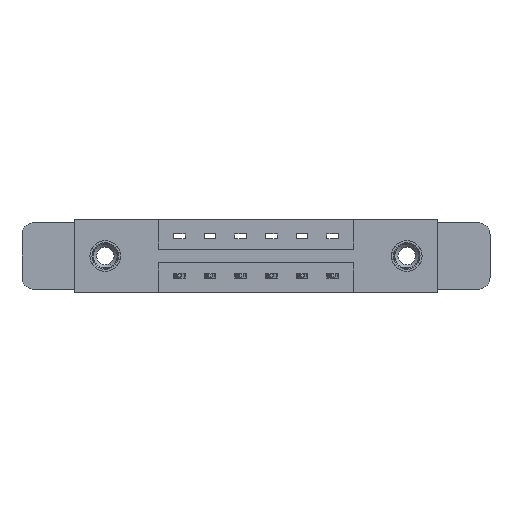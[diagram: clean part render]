
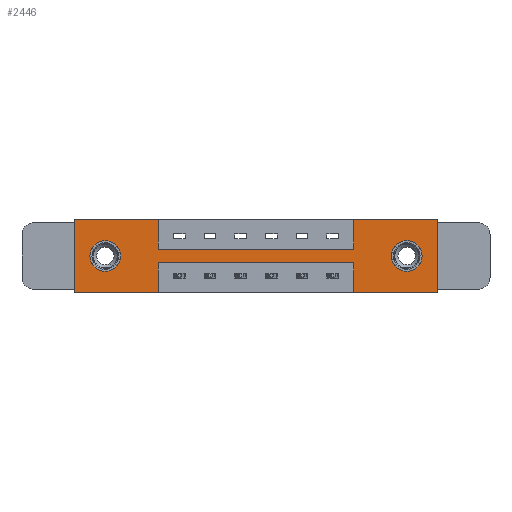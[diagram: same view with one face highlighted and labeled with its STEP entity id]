
A CAD part, front view. The second image highlights one B-rep face of the part: STEP entity #2446.
In plain terms, the highlighted planar face has unit normal (0, -1, 0).
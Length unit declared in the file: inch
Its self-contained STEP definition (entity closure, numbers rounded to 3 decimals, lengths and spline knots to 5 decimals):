
#35 = DIRECTION ( 'NONE',  ( 0., 1., 0. ) ) ;
#72 = CARTESIAN_POINT ( 'NONE',  ( 1.687, 0., -0.263 ) ) ;
#93 = ORIENTED_EDGE ( 'NONE', *, *, #8928, .F. ) ;
#447 = LINE ( 'NONE', #4689, #7954 ) ;
#464 = EDGE_CURVE ( 'NONE', #8278, #10195, #6132, .T. ) ;
#493 = CARTESIAN_POINT ( 'NONE',  ( 0.425, 0., 0. ) ) ;
#571 = CIRCLE ( 'NONE', #1085, 0.078 ) ;
#808 = LINE ( 'NONE', #3687, #4784 ) ;
#823 = ORIENTED_EDGE ( 'NONE', *, *, #11051, .F. ) ;
#857 = VERTEX_POINT ( 'NONE', #7307 ) ;
#1085 = AXIS2_PLACEMENT_3D ( 'NONE', #3840, #9292, #11082 ) ;
#1113 = CARTESIAN_POINT ( 'NONE',  ( 0., 0., 0. ) ) ;
#1230 = CARTESIAN_POINT ( 'NONE',  ( 0.155, 0., -0.107 ) ) ;
#1472 = ORIENTED_EDGE ( 'NONE', *, *, #464, .F. ) ;
#1555 = EDGE_CURVE ( 'NONE', #4462, #7166, #3856, .T. ) ;
#1600 = CARTESIAN_POINT ( 'NONE',  ( 1.417, 0., -0.15 ) ) ;
#1787 = ORIENTED_EDGE ( 'NONE', *, *, #2870, .T. ) ;
#2103 = CIRCLE ( 'NONE', #7834, 0.078 ) ;
#2293 = VECTOR ( 'NONE', #5236, 39.37008 ) ;
#2316 = CARTESIAN_POINT ( 'NONE',  ( 0.425, 0., -0.15 ) ) ;
#2446 = ADVANCED_FACE ( 'NONE', ( #9237, #8093, #8958 ), #11409, .T. ) ;
#2493 = CARTESIAN_POINT ( 'NONE',  ( 1.417, 0., -0.37 ) ) ;
#2511 = CARTESIAN_POINT ( 'NONE',  ( 0.425, 0., -0.37 ) ) ;
#2624 = EDGE_CURVE ( 'NONE', #10195, #3910, #10980, .T. ) ;
#2663 = CARTESIAN_POINT ( 'NONE',  ( 0.425, 0., 0. ) ) ;
#2870 = EDGE_CURVE ( 'NONE', #8690, #9549, #571, .T. ) ;
#2927 = VERTEX_POINT ( 'NONE', #8402 ) ;
#2949 = EDGE_LOOP ( 'NONE', ( #10601, #3054, #823, #3131, #5890, #1472, #8414, #6598, #2987, #8954, #4121, #93 ) ) ;
#2987 = ORIENTED_EDGE ( 'NONE', *, *, #10875, .F. ) ;
#3054 = ORIENTED_EDGE ( 'NONE', *, *, #5545, .F. ) ;
#3131 = ORIENTED_EDGE ( 'NONE', *, *, #8662, .F. ) ;
#3208 = DIRECTION ( 'NONE',  ( 0., 0., -1. ) ) ;
#3327 = VECTOR ( 'NONE', #5101, 39.37008 ) ;
#3341 = CARTESIAN_POINT ( 'NONE',  ( 0.425, 0., -0.37 ) ) ;
#3411 = LINE ( 'NONE', #2316, #7914 ) ;
#3439 = CARTESIAN_POINT ( 'NONE',  ( 0.425, 0., -0.15 ) ) ;
#3445 = EDGE_CURVE ( 'NONE', #4766, #3598, #3411, .T. ) ;
#3598 = VERTEX_POINT ( 'NONE', #1600 ) ;
#3615 = DIRECTION ( 'NONE',  ( 0., 0., 1. ) ) ;
#3654 = VERTEX_POINT ( 'NONE', #8764 ) ;
#3687 = CARTESIAN_POINT ( 'NONE',  ( 0.425, 0., -0.22 ) ) ;
#3840 = CARTESIAN_POINT ( 'NONE',  ( 1.687, 0., -0.185 ) ) ;
#3856 = LINE ( 'NONE', #11221, #5380 ) ;
#3910 = VERTEX_POINT ( 'NONE', #7349 ) ;
#4015 = CARTESIAN_POINT ( 'NONE',  ( 1.687, 0., -0.107 ) ) ;
#4121 = ORIENTED_EDGE ( 'NONE', *, *, #1555, .F. ) ;
#4282 = VECTOR ( 'NONE', #4962, 39.37008 ) ;
#4322 = CARTESIAN_POINT ( 'NONE',  ( 0., 0., 0. ) ) ;
#4343 = EDGE_LOOP ( 'NONE', ( #8923, #7472 ) ) ;
#4462 = VERTEX_POINT ( 'NONE', #9364 ) ;
#4470 = VERTEX_POINT ( 'NONE', #1230 ) ;
#4689 = CARTESIAN_POINT ( 'NONE',  ( 1.417, 0., 0. ) ) ;
#4701 = ORIENTED_EDGE ( 'NONE', *, *, #5756, .T. ) ;
#4766 = VERTEX_POINT ( 'NONE', #3439 ) ;
#4784 = VECTOR ( 'NONE', #6395, 39.37008 ) ;
#4912 = EDGE_LOOP ( 'NONE', ( #1787, #4701 ) ) ;
#4927 = DIRECTION ( 'NONE',  ( 0., 1., 0. ) ) ;
#4958 = VECTOR ( 'NONE', #11738, 39.37008 ) ;
#4962 = DIRECTION ( 'NONE',  ( 0., 0., -1. ) ) ;
#5101 = DIRECTION ( 'NONE',  ( 0., 0., -1. ) ) ;
#5236 = DIRECTION ( 'NONE',  ( 0., 0., 1. ) ) ;
#5293 = DIRECTION ( 'NONE',  ( 0., 1., 0. ) ) ;
#5358 = DIRECTION ( 'NONE',  ( 0., 0., 1. ) ) ;
#5380 = VECTOR ( 'NONE', #10156, 39.37008 ) ;
#5438 = CARTESIAN_POINT ( 'NONE',  ( 0., 0., -0.37 ) ) ;
#5545 = EDGE_CURVE ( 'NONE', #857, #2927, #808, .T. ) ;
#5616 = VERTEX_POINT ( 'NONE', #2663 ) ;
#5634 = EDGE_CURVE ( 'NONE', #7166, #5616, #11198, .T. ) ;
#5756 = EDGE_CURVE ( 'NONE', #9549, #8690, #8302, .T. ) ;
#5772 = AXIS2_PLACEMENT_3D ( 'NONE', #7779, #7730, #3208 ) ;
#5889 = DIRECTION ( 'NONE',  ( 1., 0., 0. ) ) ;
#5890 = ORIENTED_EDGE ( 'NONE', *, *, #2624, .F. ) ;
#6092 = DIRECTION ( 'NONE',  ( 1., 0., 0. ) ) ;
#6132 = LINE ( 'NONE', #1113, #7980 ) ;
#6280 = CARTESIAN_POINT ( 'NONE',  ( 1.417, 0., -0.37 ) ) ;
#6395 = DIRECTION ( 'NONE',  ( -1., 0., 0. ) ) ;
#6598 = ORIENTED_EDGE ( 'NONE', *, *, #3445, .F. ) ;
#6727 = VECTOR ( 'NONE', #9914, 39.37008 ) ;
#6730 = DIRECTION ( 'NONE',  ( 0., 0., -1. ) ) ;
#6945 = DIRECTION ( 'NONE',  ( 0., 0., -1. ) ) ;
#6949 = VECTOR ( 'NONE', #8556, 39.37008 ) ;
#7071 = CARTESIAN_POINT ( 'NONE',  ( 0.155, 0., -0.185 ) ) ;
#7165 = EDGE_CURVE ( 'NONE', #2927, #7195, #10871, .T. ) ;
#7166 = VERTEX_POINT ( 'NONE', #4322 ) ;
#7195 = VERTEX_POINT ( 'NONE', #3341 ) ;
#7307 = CARTESIAN_POINT ( 'NONE',  ( 1.417, 0., -0.22 ) ) ;
#7349 = CARTESIAN_POINT ( 'NONE',  ( 1.842, 0., -0.37 ) ) ;
#7472 = ORIENTED_EDGE ( 'NONE', *, *, #8976, .T. ) ;
#7638 = CIRCLE ( 'NONE', #10293, 0.078 ) ;
#7730 = DIRECTION ( 'NONE',  ( 0., -1., 0. ) ) ;
#7779 = CARTESIAN_POINT ( 'NONE',  ( 0., 0., -0.37 ) ) ;
#7834 = AXIS2_PLACEMENT_3D ( 'NONE', #9835, #35, #5358 ) ;
#7914 = VECTOR ( 'NONE', #5889, 39.37008 ) ;
#7954 = VECTOR ( 'NONE', #11074, 39.37008 ) ;
#7980 = VECTOR ( 'NONE', #6092, 39.37008 ) ;
#8091 = CARTESIAN_POINT ( 'NONE',  ( 1.417, 0., 0. ) ) ;
#8093 = FACE_BOUND ( 'NONE', #4343, .T. ) ;
#8278 = VERTEX_POINT ( 'NONE', #8091 ) ;
#8302 = CIRCLE ( 'NONE', #9651, 0.078 ) ;
#8402 = CARTESIAN_POINT ( 'NONE',  ( 0.425, 0., -0.22 ) ) ;
#8414 = ORIENTED_EDGE ( 'NONE', *, *, #8456, .F. ) ;
#8456 = EDGE_CURVE ( 'NONE', #3598, #8278, #447, .T. ) ;
#8556 = DIRECTION ( 'NONE',  ( -1., 0., 0. ) ) ;
#8582 = CARTESIAN_POINT ( 'NONE',  ( 1.842, 0., 0. ) ) ;
#8652 = LINE ( 'NONE', #5438, #4958 ) ;
#8662 = EDGE_CURVE ( 'NONE', #3910, #9005, #10377, .T. ) ;
#8690 = VERTEX_POINT ( 'NONE', #4015 ) ;
#8764 = CARTESIAN_POINT ( 'NONE',  ( 0.155, 0., -0.263 ) ) ;
#8923 = ORIENTED_EDGE ( 'NONE', *, *, #9440, .T. ) ;
#8928 = EDGE_CURVE ( 'NONE', #7195, #4462, #8652, .T. ) ;
#8945 = VECTOR ( 'NONE', #6945, 39.37008 ) ;
#8954 = ORIENTED_EDGE ( 'NONE', *, *, #5634, .F. ) ;
#8958 = FACE_OUTER_BOUND ( 'NONE', #2949, .T. ) ;
#8964 = LINE ( 'NONE', #493, #4282 ) ;
#8976 = EDGE_CURVE ( 'NONE', #3654, #4470, #7638, .T. ) ;
#9005 = VERTEX_POINT ( 'NONE', #6280 ) ;
#9237 = FACE_BOUND ( 'NONE', #4912, .T. ) ;
#9292 = DIRECTION ( 'NONE',  ( 0., 1., 0. ) ) ;
#9364 = CARTESIAN_POINT ( 'NONE',  ( 0., 0., -0.37 ) ) ;
#9440 = EDGE_CURVE ( 'NONE', #4470, #3654, #2103, .T. ) ;
#9549 = VERTEX_POINT ( 'NONE', #72 ) ;
#9651 = AXIS2_PLACEMENT_3D ( 'NONE', #11363, #4927, #6730 ) ;
#9739 = CARTESIAN_POINT ( 'NONE',  ( 1.842, 0., 0. ) ) ;
#9835 = CARTESIAN_POINT ( 'NONE',  ( 0.155, 0., -0.185 ) ) ;
#9914 = DIRECTION ( 'NONE',  ( 1., 0., 0. ) ) ;
#9959 = CARTESIAN_POINT ( 'NONE',  ( 0., 0., 0. ) ) ;
#10156 = DIRECTION ( 'NONE',  ( 0., 0., 1. ) ) ;
#10195 = VERTEX_POINT ( 'NONE', #8582 ) ;
#10293 = AXIS2_PLACEMENT_3D ( 'NONE', #7071, #5293, #3615 ) ;
#10377 = LINE ( 'NONE', #10487, #6949 ) ;
#10487 = CARTESIAN_POINT ( 'NONE',  ( 0., 0., -0.37 ) ) ;
#10601 = ORIENTED_EDGE ( 'NONE', *, *, #7165, .F. ) ;
#10871 = LINE ( 'NONE', #2511, #3327 ) ;
#10875 = EDGE_CURVE ( 'NONE', #5616, #4766, #8964, .T. ) ;
#10980 = LINE ( 'NONE', #9739, #8945 ) ;
#11051 = EDGE_CURVE ( 'NONE', #9005, #857, #11116, .T. ) ;
#11074 = DIRECTION ( 'NONE',  ( 0., 0., 1. ) ) ;
#11082 = DIRECTION ( 'NONE',  ( 0., 0., -1. ) ) ;
#11116 = LINE ( 'NONE', #2493, #2293 ) ;
#11198 = LINE ( 'NONE', #9959, #6727 ) ;
#11221 = CARTESIAN_POINT ( 'NONE',  ( 0., 0., 0. ) ) ;
#11363 = CARTESIAN_POINT ( 'NONE',  ( 1.687, 0., -0.185 ) ) ;
#11409 = PLANE ( 'NONE',  #5772 ) ;
#11738 = DIRECTION ( 'NONE',  ( -1., 0., 0. ) ) ;
